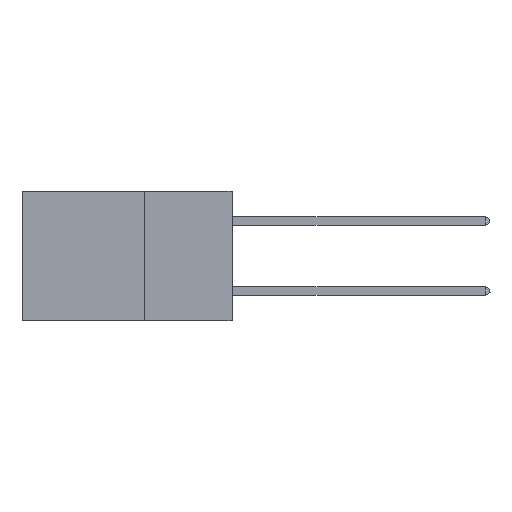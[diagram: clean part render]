
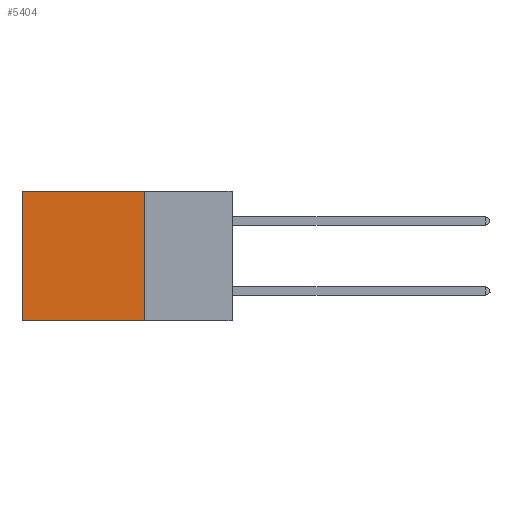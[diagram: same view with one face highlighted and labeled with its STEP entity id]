
A CAD part, left-side view. The second image highlights one B-rep face of the part: STEP entity #5404.
In plain terms, the highlighted planar face has unit normal (-1, 0, 0).
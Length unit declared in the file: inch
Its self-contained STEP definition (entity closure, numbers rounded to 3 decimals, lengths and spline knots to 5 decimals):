
#300 = CARTESIAN_POINT ( 'NONE',  ( 0.2875, 0.25, 0. ) ) ;
#1549 = DIRECTION ( 'NONE',  ( 0., 1., 0. ) ) ;
#3493 = VECTOR ( 'NONE', #1549, 39.37008 ) ;
#3820 = CARTESIAN_POINT ( 'NONE',  ( 0.2875, 0.25, 0. ) ) ;
#3921 = ORIENTED_EDGE ( 'NONE', *, *, #24661, .T. ) ;
#3971 = VECTOR ( 'NONE', #14214, 39.37008 ) ;
#4232 = CARTESIAN_POINT ( 'NONE',  ( 0.2875, 0.6, 0. ) ) ;
#4510 = CARTESIAN_POINT ( 'NONE',  ( 0.2875, 0.25, 0. ) ) ;
#4763 = VERTEX_POINT ( 'NONE', #4510 ) ;
#5404 = ADVANCED_FACE ( 'NONE', ( #5859 ), #10146, .F. ) ;
#5410 = VERTEX_POINT ( 'NONE', #21877 ) ;
#5859 = FACE_OUTER_BOUND ( 'NONE', #13791, .T. ) ;
#7862 = AXIS2_PLACEMENT_3D ( 'NONE', #300, #15044, #14845 ) ;
#8182 = VECTOR ( 'NONE', #9087, 39.37008 ) ;
#8391 = VERTEX_POINT ( 'NONE', #10902 ) ;
#8654 = DIRECTION ( 'NONE',  ( 0., 0., -1. ) ) ;
#9087 = DIRECTION ( 'NONE',  ( 0., 0., -1. ) ) ;
#9420 = CARTESIAN_POINT ( 'NONE',  ( 0.2875, 0.25, -0.37 ) ) ;
#10146 = PLANE ( 'NONE',  #7862 ) ;
#10336 = LINE ( 'NONE', #9420, #3971 ) ;
#10902 = CARTESIAN_POINT ( 'NONE',  ( 0.2875, 0.6, 0. ) ) ;
#11076 = EDGE_CURVE ( 'NONE', #4763, #8391, #21135, .T. ) ;
#11191 = EDGE_CURVE ( 'NONE', #4763, #5410, #12868, .T. ) ;
#12868 = LINE ( 'NONE', #3820, #16962 ) ;
#13791 = EDGE_LOOP ( 'NONE', ( #3921, #15886, #26407, #24984 ) ) ;
#14214 = DIRECTION ( 'NONE',  ( 0., 1., 0. ) ) ;
#14845 = DIRECTION ( 'NONE',  ( 0., 0., -1. ) ) ;
#15044 = DIRECTION ( 'NONE',  ( 1., 0., 0. ) ) ;
#15886 = ORIENTED_EDGE ( 'NONE', *, *, #16844, .F. ) ;
#16844 = EDGE_CURVE ( 'NONE', #5410, #23653, #10336, .T. ) ;
#16962 = VECTOR ( 'NONE', #8654, 39.37008 ) ;
#21135 = LINE ( 'NONE', #29740, #3493 ) ;
#21656 = CARTESIAN_POINT ( 'NONE',  ( 0.2875, 0.6, -0.37 ) ) ;
#21877 = CARTESIAN_POINT ( 'NONE',  ( 0.2875, 0.25, -0.37 ) ) ;
#23653 = VERTEX_POINT ( 'NONE', #21656 ) ;
#24661 = EDGE_CURVE ( 'NONE', #8391, #23653, #29963, .T. ) ;
#24984 = ORIENTED_EDGE ( 'NONE', *, *, #11076, .T. ) ;
#26407 = ORIENTED_EDGE ( 'NONE', *, *, #11191, .F. ) ;
#29740 = CARTESIAN_POINT ( 'NONE',  ( 0.2875, 0.25, 0. ) ) ;
#29963 = LINE ( 'NONE', #4232, #8182 ) ;
